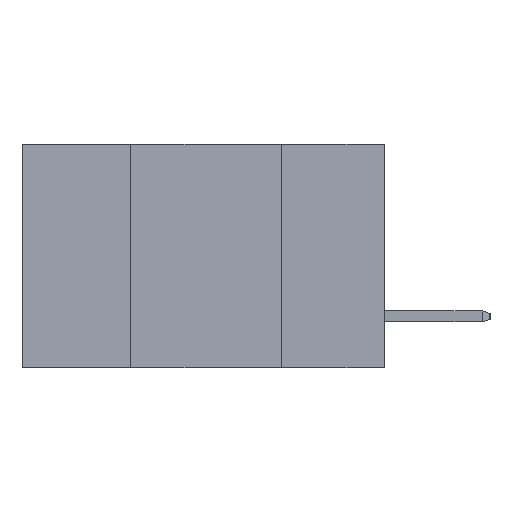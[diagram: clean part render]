
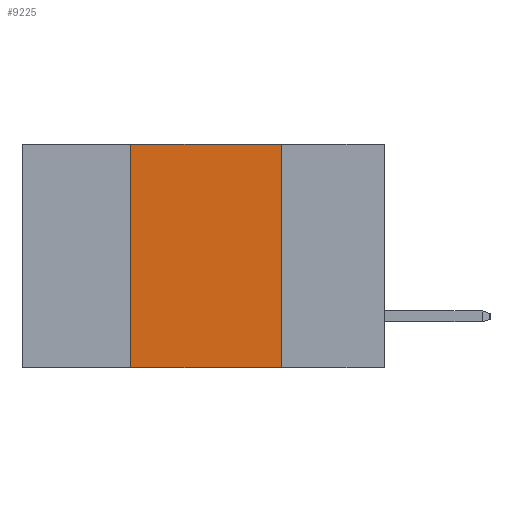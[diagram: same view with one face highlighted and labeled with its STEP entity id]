
A CAD part, left-side view. The second image highlights one B-rep face of the part: STEP entity #9225.
In plain terms, the highlighted planar face has unit normal (-1, 0, 0).
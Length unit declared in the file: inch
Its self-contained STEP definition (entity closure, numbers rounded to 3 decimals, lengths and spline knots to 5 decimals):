
#145 = CARTESIAN_POINT ( 'NONE',  ( 0., 0.6, 0. ) ) ;
#383 = DIRECTION ( 'NONE',  ( 0., -1., 0. ) ) ;
#584 = ORIENTED_EDGE ( 'NONE', *, *, #9776, .F. ) ;
#617 = EDGE_CURVE ( 'NONE', #12060, #6212, #12378, .T. ) ;
#1136 = ORIENTED_EDGE ( 'NONE', *, *, #617, .F. ) ;
#1664 = VECTOR ( 'NONE', #13592, 39.37008 ) ;
#2004 = CARTESIAN_POINT ( 'NONE',  ( 0., 0.17, 0. ) ) ;
#2184 = CARTESIAN_POINT ( 'NONE',  ( 0., 0.42, -0.37 ) ) ;
#2442 = EDGE_CURVE ( 'NONE', #12839, #12313, #4597, .T. ) ;
#2523 = DIRECTION ( 'NONE',  ( 0., 0., -1. ) ) ;
#2681 = AXIS2_PLACEMENT_3D ( 'NONE', #145, #8925, #2523 ) ;
#3246 = CARTESIAN_POINT ( 'NONE',  ( 0., 0.42, 0. ) ) ;
#3515 = CARTESIAN_POINT ( 'NONE',  ( 0., 0.6, 0. ) ) ;
#3643 = LINE ( 'NONE', #3515, #9016 ) ;
#3734 = CARTESIAN_POINT ( 'NONE',  ( 0., 0.6, -0.37 ) ) ;
#4597 = LINE ( 'NONE', #13607, #1664 ) ;
#4628 = DIRECTION ( 'NONE',  ( 0., -1., 0. ) ) ;
#5747 = FACE_OUTER_BOUND ( 'NONE', #10779, .T. ) ;
#6212 = VERTEX_POINT ( 'NONE', #8538 ) ;
#6982 = LINE ( 'NONE', #3734, #12294 ) ;
#7000 = DIRECTION ( 'NONE',  ( 0., 0., 1. ) ) ;
#7078 = VECTOR ( 'NONE', #7000, 39.37008 ) ;
#7754 = EDGE_CURVE ( 'NONE', #12060, #12313, #6982, .T. ) ;
#8538 = CARTESIAN_POINT ( 'NONE',  ( 0., 0.42, 0. ) ) ;
#8925 = DIRECTION ( 'NONE',  ( 1., 0., 0. ) ) ;
#9016 = VECTOR ( 'NONE', #4628, 39.37008 ) ;
#9225 = ADVANCED_FACE ( 'NONE', ( #5747 ), #12825, .F. ) ;
#9776 = EDGE_CURVE ( 'NONE', #6212, #12839, #3643, .T. ) ;
#10251 = ORIENTED_EDGE ( 'NONE', *, *, #7754, .T. ) ;
#10779 = EDGE_LOOP ( 'NONE', ( #11154, #584, #1136, #10251 ) ) ;
#11154 = ORIENTED_EDGE ( 'NONE', *, *, #2442, .F. ) ;
#11902 = CARTESIAN_POINT ( 'NONE',  ( 0., 0.17, -0.37 ) ) ;
#12060 = VERTEX_POINT ( 'NONE', #2184 ) ;
#12294 = VECTOR ( 'NONE', #383, 39.37008 ) ;
#12313 = VERTEX_POINT ( 'NONE', #11902 ) ;
#12378 = LINE ( 'NONE', #3246, #7078 ) ;
#12825 = PLANE ( 'NONE',  #2681 ) ;
#12839 = VERTEX_POINT ( 'NONE', #2004 ) ;
#13592 = DIRECTION ( 'NONE',  ( 0., 0., -1. ) ) ;
#13607 = CARTESIAN_POINT ( 'NONE',  ( 0., 0.17, 0. ) ) ;
